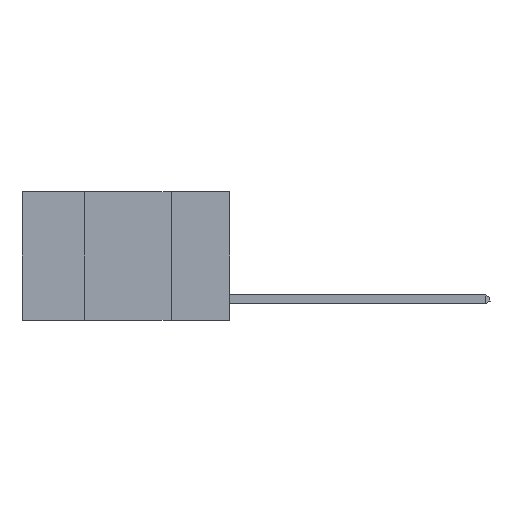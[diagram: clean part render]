
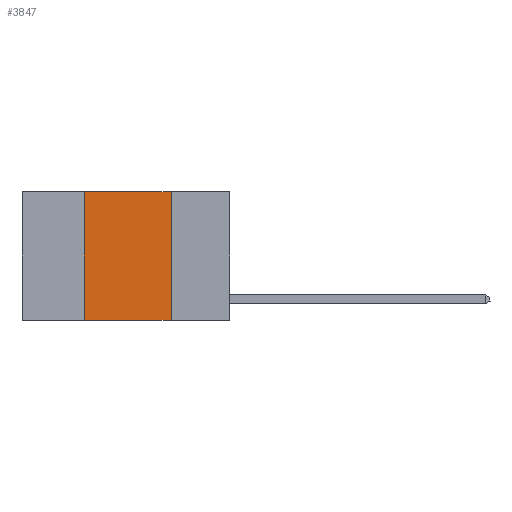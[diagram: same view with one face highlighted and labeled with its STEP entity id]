
A CAD part, left-side view. The second image highlights one B-rep face of the part: STEP entity #3847.
In plain terms, the highlighted planar face has unit normal (-1, 0, 0).
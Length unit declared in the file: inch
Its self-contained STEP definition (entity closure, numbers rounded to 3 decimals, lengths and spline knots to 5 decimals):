
#273 = DIRECTION ( 'NONE',  ( 0., 0., -1. ) ) ;
#411 = VECTOR ( 'NONE', #894, 39.37008 ) ;
#856 = CARTESIAN_POINT ( 'NONE',  ( 0., 0.6, -0.37 ) ) ;
#894 = DIRECTION ( 'NONE',  ( 0., -1., 0. ) ) ;
#989 = CARTESIAN_POINT ( 'NONE',  ( 0., 0.42, 0. ) ) ;
#1009 = EDGE_CURVE ( 'NONE', #5497, #6071, #5274, .T. ) ;
#1133 = VERTEX_POINT ( 'NONE', #4023 ) ;
#1202 = CARTESIAN_POINT ( 'NONE',  ( 0., 0.6, 0. ) ) ;
#1297 = VECTOR ( 'NONE', #7900, 39.37008 ) ;
#2158 = LINE ( 'NONE', #856, #411 ) ;
#2626 = CARTESIAN_POINT ( 'NONE',  ( 0., 0.17, 0. ) ) ;
#3451 = CARTESIAN_POINT ( 'NONE',  ( 0., 0.17, -0.37 ) ) ;
#3797 = EDGE_CURVE ( 'NONE', #1133, #6071, #2158, .T. ) ;
#3847 = ADVANCED_FACE ( 'NONE', ( #6948 ), #6306, .F. ) ;
#4023 = CARTESIAN_POINT ( 'NONE',  ( 0., 0.42, -0.37 ) ) ;
#4336 = AXIS2_PLACEMENT_3D ( 'NONE', #5510, #7528, #273 ) ;
#4413 = LINE ( 'NONE', #989, #5419 ) ;
#5042 = VECTOR ( 'NONE', #6547, 39.37008 ) ;
#5274 = LINE ( 'NONE', #2626, #1297 ) ;
#5419 = VECTOR ( 'NONE', #8216, 39.37008 ) ;
#5497 = VERTEX_POINT ( 'NONE', #8058 ) ;
#5510 = CARTESIAN_POINT ( 'NONE',  ( 0., 0.6, 0. ) ) ;
#5737 = ORIENTED_EDGE ( 'NONE', *, *, #6752, .F. ) ;
#5895 = CARTESIAN_POINT ( 'NONE',  ( 0., 0.42, 0. ) ) ;
#5983 = LINE ( 'NONE', #1202, #5042 ) ;
#6071 = VERTEX_POINT ( 'NONE', #3451 ) ;
#6259 = ORIENTED_EDGE ( 'NONE', *, *, #3797, .T. ) ;
#6306 = PLANE ( 'NONE',  #4336 ) ;
#6547 = DIRECTION ( 'NONE',  ( 0., -1., 0. ) ) ;
#6752 = EDGE_CURVE ( 'NONE', #7316, #5497, #5983, .T. ) ;
#6834 = ORIENTED_EDGE ( 'NONE', *, *, #1009, .F. ) ;
#6948 = FACE_OUTER_BOUND ( 'NONE', #7998, .T. ) ;
#7316 = VERTEX_POINT ( 'NONE', #5895 ) ;
#7432 = ORIENTED_EDGE ( 'NONE', *, *, #7831, .F. ) ;
#7528 = DIRECTION ( 'NONE',  ( 1., 0., 0. ) ) ;
#7831 = EDGE_CURVE ( 'NONE', #1133, #7316, #4413, .T. ) ;
#7900 = DIRECTION ( 'NONE',  ( 0., 0., -1. ) ) ;
#7998 = EDGE_LOOP ( 'NONE', ( #6834, #5737, #7432, #6259 ) ) ;
#8058 = CARTESIAN_POINT ( 'NONE',  ( 0., 0.17, 0. ) ) ;
#8216 = DIRECTION ( 'NONE',  ( 0., 0., 1. ) ) ;
